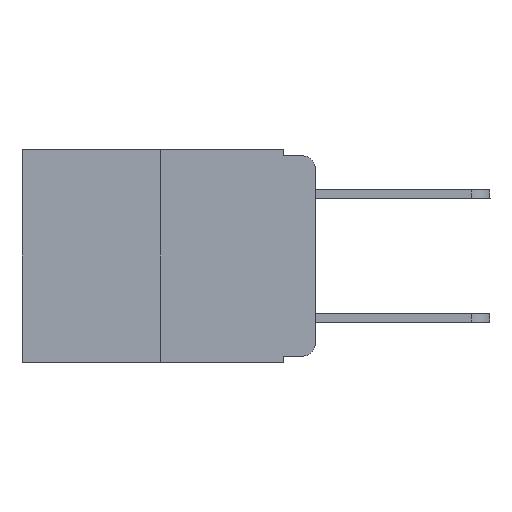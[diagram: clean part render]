
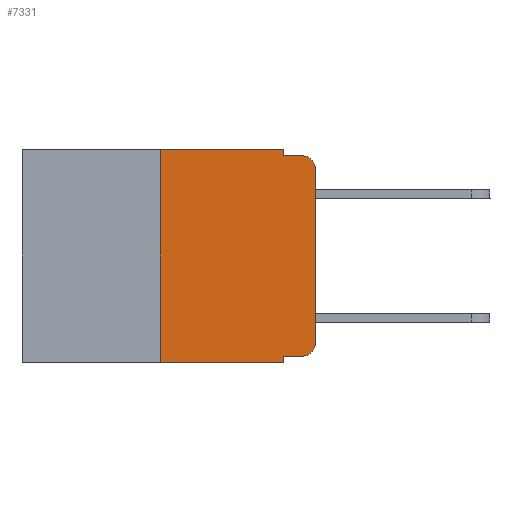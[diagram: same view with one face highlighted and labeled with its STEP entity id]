
A CAD part, left-side view. The second image highlights one B-rep face of the part: STEP entity #7331.
In plain terms, the highlighted planar face has unit normal (-1, 0, 0).
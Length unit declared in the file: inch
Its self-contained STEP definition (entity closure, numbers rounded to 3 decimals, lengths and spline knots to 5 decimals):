
#2 = VERTEX_POINT ( 'NONE', #4307 ) ;
#70 = CARTESIAN_POINT ( 'NONE',  ( 0., 0., -0.03 ) ) ;
#231 = LINE ( 'NONE', #1734, #3830 ) ;
#313 = EDGE_CURVE ( 'NONE', #16574, #16048, #11673, .T. ) ;
#552 = EDGE_CURVE ( 'NONE', #2103, #5376, #4237, .T. ) ;
#569 = VECTOR ( 'NONE', #14084, 39.37008 ) ;
#958 = DIRECTION ( 'NONE',  ( 0., 0., 1. ) ) ;
#1305 = VERTEX_POINT ( 'NONE', #6277 ) ;
#1417 = AXIS2_PLACEMENT_3D ( 'NONE', #2293, #15198, #18019 ) ;
#1611 = ORIENTED_EDGE ( 'NONE', *, *, #12325, .T. ) ;
#1734 = CARTESIAN_POINT ( 'NONE',  ( 0., 0.051, 0. ) ) ;
#2103 = VERTEX_POINT ( 'NONE', #70 ) ;
#2139 = CARTESIAN_POINT ( 'NONE',  ( 0., 0.25, 0. ) ) ;
#2221 = CARTESIAN_POINT ( 'NONE',  ( 0., 0.051, -0.333 ) ) ;
#2293 = CARTESIAN_POINT ( 'NONE',  ( 0., 0.473, 0. ) ) ;
#3164 = EDGE_CURVE ( 'NONE', #5708, #2103, #9355, .T. ) ;
#3382 = VECTOR ( 'NONE', #958, 39.37008 ) ;
#3581 = CARTESIAN_POINT ( 'NONE',  ( 0., 0.02, -0.03 ) ) ;
#3644 = LINE ( 'NONE', #2221, #17479 ) ;
#3789 = CARTESIAN_POINT ( 'NONE',  ( 0., 0., 0. ) ) ;
#3830 = VECTOR ( 'NONE', #17844, 39.37008 ) ;
#4237 = CIRCLE ( 'NONE', #14778, 0.02 ) ;
#4307 = CARTESIAN_POINT ( 'NONE',  ( 0., 0.051, 0. ) ) ;
#4483 = VERTEX_POINT ( 'NONE', #14719 ) ;
#4719 = DIRECTION ( 'NONE',  ( 0., 0., -1. ) ) ;
#4894 = LINE ( 'NONE', #2139, #5075 ) ;
#4963 = ORIENTED_EDGE ( 'NONE', *, *, #313, .T. ) ;
#5049 = LINE ( 'NONE', #7693, #17337 ) ;
#5075 = VECTOR ( 'NONE', #17879, 39.37008 ) ;
#5230 = DIRECTION ( 'NONE',  ( 0., -1., 0. ) ) ;
#5376 = VERTEX_POINT ( 'NONE', #18607 ) ;
#5393 = DIRECTION ( 'NONE',  ( 0., 0., -1. ) ) ;
#5640 = EDGE_CURVE ( 'NONE', #4483, #5376, #9655, .T. ) ;
#5708 = VERTEX_POINT ( 'NONE', #7198 ) ;
#5925 = CIRCLE ( 'NONE', #15262, 0.02 ) ;
#6066 = ORIENTED_EDGE ( 'NONE', *, *, #3164, .T. ) ;
#6277 = CARTESIAN_POINT ( 'NONE',  ( 0., 0.051, -0.333 ) ) ;
#6967 = EDGE_CURVE ( 'NONE', #1305, #13730, #3644, .T. ) ;
#7198 = CARTESIAN_POINT ( 'NONE',  ( 0., 0., -0.313 ) ) ;
#7206 = VERTEX_POINT ( 'NONE', #11905 ) ;
#7292 = DIRECTION ( 'NONE',  ( 0., -1., 0. ) ) ;
#7331 = ADVANCED_FACE ( 'NONE', ( #18111 ), #15297, .F. ) ;
#7425 = CARTESIAN_POINT ( 'NONE',  ( 0., 0.02, -0.333 ) ) ;
#7533 = ORIENTED_EDGE ( 'NONE', *, *, #13838, .F. ) ;
#7693 = CARTESIAN_POINT ( 'NONE',  ( 0., 0.051, 0. ) ) ;
#8458 = ORIENTED_EDGE ( 'NONE', *, *, #6967, .T. ) ;
#8965 = ORIENTED_EDGE ( 'NONE', *, *, #17381, .F. ) ;
#9355 = LINE ( 'NONE', #3789, #3382 ) ;
#9655 = LINE ( 'NONE', #15401, #569 ) ;
#9912 = ORIENTED_EDGE ( 'NONE', *, *, #11705, .F. ) ;
#10068 = ORIENTED_EDGE ( 'NONE', *, *, #5640, .F. ) ;
#10537 = ORIENTED_EDGE ( 'NONE', *, *, #552, .T. ) ;
#10907 = CARTESIAN_POINT ( 'NONE',  ( 0., 0.25, -0.343 ) ) ;
#11528 = CARTESIAN_POINT ( 'NONE',  ( 0., 0.051, -0.343 ) ) ;
#11673 = LINE ( 'NONE', #17420, #14465 ) ;
#11705 = EDGE_CURVE ( 'NONE', #1305, #16048, #5049, .T. ) ;
#11862 = DIRECTION ( 'NONE',  ( -1., 0., 0. ) ) ;
#11905 = CARTESIAN_POINT ( 'NONE',  ( 0., 0.25, 0. ) ) ;
#12180 = EDGE_CURVE ( 'NONE', #2, #4483, #231, .T. ) ;
#12325 = EDGE_CURVE ( 'NONE', #13730, #5708, #5925, .T. ) ;
#12781 = EDGE_LOOP ( 'NONE', ( #6066, #10537, #10068, #17892, #8965, #7533, #4963, #9912, #8458, #1611 ) ) ;
#13730 = VERTEX_POINT ( 'NONE', #7425 ) ;
#13787 = CARTESIAN_POINT ( 'NONE',  ( 0., 0.02, -0.313 ) ) ;
#13838 = EDGE_CURVE ( 'NONE', #16574, #7206, #4894, .T. ) ;
#14084 = DIRECTION ( 'NONE',  ( 0., -1., 0. ) ) ;
#14453 = CARTESIAN_POINT ( 'NONE',  ( 0., 0.473, 0. ) ) ;
#14465 = VECTOR ( 'NONE', #14609, 39.37008 ) ;
#14609 = DIRECTION ( 'NONE',  ( 0., -1., 0. ) ) ;
#14719 = CARTESIAN_POINT ( 'NONE',  ( 0., 0.051, -0.01 ) ) ;
#14772 = VECTOR ( 'NONE', #7292, 39.37008 ) ;
#14778 = AXIS2_PLACEMENT_3D ( 'NONE', #3581, #11862, #4719 ) ;
#14839 = LINE ( 'NONE', #14453, #14772 ) ;
#15114 = DIRECTION ( 'NONE',  ( -1., 0., 0. ) ) ;
#15198 = DIRECTION ( 'NONE',  ( 1., 0., 0. ) ) ;
#15262 = AXIS2_PLACEMENT_3D ( 'NONE', #13787, #15114, #5393 ) ;
#15297 = PLANE ( 'NONE',  #1417 ) ;
#15401 = CARTESIAN_POINT ( 'NONE',  ( 0., 0.051, -0.01 ) ) ;
#16048 = VERTEX_POINT ( 'NONE', #11528 ) ;
#16574 = VERTEX_POINT ( 'NONE', #10907 ) ;
#17337 = VECTOR ( 'NONE', #17584, 39.37008 ) ;
#17381 = EDGE_CURVE ( 'NONE', #7206, #2, #14839, .T. ) ;
#17420 = CARTESIAN_POINT ( 'NONE',  ( 0., 0.473, -0.343 ) ) ;
#17479 = VECTOR ( 'NONE', #5230, 39.37008 ) ;
#17584 = DIRECTION ( 'NONE',  ( 0., 0., -1. ) ) ;
#17844 = DIRECTION ( 'NONE',  ( 0., 0., -1. ) ) ;
#17879 = DIRECTION ( 'NONE',  ( 0., 0., 1. ) ) ;
#17892 = ORIENTED_EDGE ( 'NONE', *, *, #12180, .F. ) ;
#18019 = DIRECTION ( 'NONE',  ( 0., 0., -1. ) ) ;
#18111 = FACE_OUTER_BOUND ( 'NONE', #12781, .T. ) ;
#18607 = CARTESIAN_POINT ( 'NONE',  ( 0., 0.02, -0.01 ) ) ;
